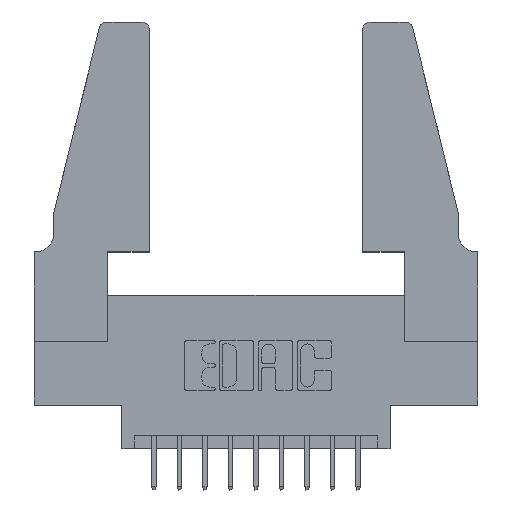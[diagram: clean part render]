
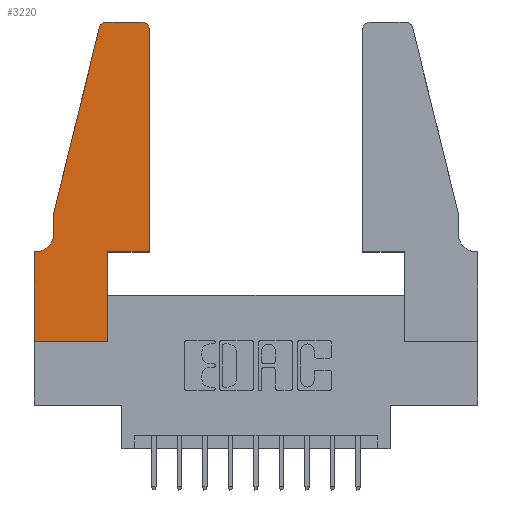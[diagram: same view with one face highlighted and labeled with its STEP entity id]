
A CAD part, top view. The second image highlights one B-rep face of the part: STEP entity #3220.
In plain terms, the highlighted planar face has unit normal (0, 0, 1).
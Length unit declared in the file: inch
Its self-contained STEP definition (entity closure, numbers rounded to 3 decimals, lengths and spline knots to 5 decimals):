
#200 = DIRECTION ( 'NONE',  ( 1., 0., 0. ) ) ;
#277 = VERTEX_POINT ( 'NONE', #6747 ) ;
#417 = LINE ( 'NONE', #4542, #11494 ) ;
#638 = CARTESIAN_POINT ( 'NONE',  ( 0.284, 1.25, 0.37 ) ) ;
#674 = VERTEX_POINT ( 'NONE', #3287 ) ;
#697 = EDGE_CURVE ( 'NONE', #674, #277, #417, .T. ) ;
#791 = DIRECTION ( 'NONE',  ( 1., 0., 0. ) ) ;
#899 = EDGE_CURVE ( 'NONE', #1029, #11434, #8804, .T. ) ;
#903 = CARTESIAN_POINT ( 'NONE',  ( 0.4205, 1.25, 0.37 ) ) ;
#1025 = DIRECTION ( 'NONE',  ( 0., 0., 1. ) ) ;
#1029 = VERTEX_POINT ( 'NONE', #6420 ) ;
#1111 = AXIS2_PLACEMENT_3D ( 'NONE', #13665, #13468, #5983 ) ;
#1183 = ORIENTED_EDGE ( 'NONE', *, *, #4739, .T. ) ;
#1201 = ORIENTED_EDGE ( 'NONE', *, *, #9031, .T. ) ;
#1419 = VECTOR ( 'NONE', #8248, 39.37008 ) ;
#1561 = EDGE_CURVE ( 'NONE', #5994, #674, #5780, .T. ) ;
#1776 = CARTESIAN_POINT ( 'NONE',  ( 0.4505, 0.35, 0.37 ) ) ;
#1813 = CARTESIAN_POINT ( 'NONE',  ( 0.2865, 0.35, 0.37 ) ) ;
#1864 = DIRECTION ( 'NONE',  ( 1., 0., 0. ) ) ;
#2030 = ORIENTED_EDGE ( 'NONE', *, *, #11785, .T. ) ;
#2249 = CARTESIAN_POINT ( 'NONE',  ( 0.284, 1.22, 0.37 ) ) ;
#2263 = CARTESIAN_POINT ( 'NONE',  ( 0.0755, 0.5, 0.37 ) ) ;
#2350 = CARTESIAN_POINT ( 'NONE',  ( 0., 0., 0.37 ) ) ;
#2599 = VECTOR ( 'NONE', #791, 39.37008 ) ;
#2892 = VECTOR ( 'NONE', #11044, 39.37008 ) ;
#2911 = ORIENTED_EDGE ( 'NONE', *, *, #1561, .T. ) ;
#3055 = EDGE_CURVE ( 'NONE', #13741, #5382, #11149, .T. ) ;
#3220 = ADVANCED_FACE ( 'NONE', ( #8140 ), #6419, .T. ) ;
#3287 = CARTESIAN_POINT ( 'NONE',  ( 0., 0.35, 0.37 ) ) ;
#3432 = LINE ( 'NONE', #2263, #13652 ) ;
#3437 = AXIS2_PLACEMENT_3D ( 'NONE', #12783, #1025, #6462 ) ;
#3440 = LINE ( 'NONE', #1813, #1419 ) ;
#3792 = ORIENTED_EDGE ( 'NONE', *, *, #697, .T. ) ;
#3890 = CARTESIAN_POINT ( 'NONE',  ( 0.4505, 1.22, 0.37 ) ) ;
#4404 = CARTESIAN_POINT ( 'NONE',  ( 0.0755, 0.5, 0.37 ) ) ;
#4542 = CARTESIAN_POINT ( 'NONE',  ( 0., 0., 0.37 ) ) ;
#4690 = CARTESIAN_POINT ( 'NONE',  ( 0.25487, 1.22718, 0.37 ) ) ;
#4714 = CARTESIAN_POINT ( 'NONE',  ( 0.2865, 0., 0.37 ) ) ;
#4722 = VERTEX_POINT ( 'NONE', #903 ) ;
#4739 = EDGE_CURVE ( 'NONE', #8224, #5994, #10923, .T. ) ;
#4751 = CARTESIAN_POINT ( 'NONE',  ( 0.0755, 0.35, 0.37 ) ) ;
#5096 = ORIENTED_EDGE ( 'NONE', *, *, #7326, .T. ) ;
#5260 = VECTOR ( 'NONE', #10212, 39.37008 ) ;
#5294 = VERTEX_POINT ( 'NONE', #638 ) ;
#5382 = VERTEX_POINT ( 'NONE', #6079 ) ;
#5386 = ORIENTED_EDGE ( 'NONE', *, *, #8547, .T. ) ;
#5539 = DIRECTION ( 'NONE',  ( 0., -1., 0. ) ) ;
#5780 = LINE ( 'NONE', #4751, #5260 ) ;
#5925 = CARTESIAN_POINT ( 'NONE',  ( 0.0055, 0.35, 0.37 ) ) ;
#5983 = DIRECTION ( 'NONE',  ( -1., 0., 0. ) ) ;
#5994 = VERTEX_POINT ( 'NONE', #5925 ) ;
#6079 = CARTESIAN_POINT ( 'NONE',  ( 0.0755, 0.5, 0.37 ) ) ;
#6184 = VERTEX_POINT ( 'NONE', #4714 ) ;
#6419 = PLANE ( 'NONE',  #3437 ) ;
#6420 = CARTESIAN_POINT ( 'NONE',  ( 0.2865, 0.35, 0.37 ) ) ;
#6462 = DIRECTION ( 'NONE',  ( 1., 0., 0. ) ) ;
#6649 = DIRECTION ( 'NONE',  ( 1., 0., 0. ) ) ;
#6671 = ORIENTED_EDGE ( 'NONE', *, *, #13728, .T. ) ;
#6747 = CARTESIAN_POINT ( 'NONE',  ( 0., 0., 0.37 ) ) ;
#6778 = CIRCLE ( 'NONE', #12624, 0.03 ) ;
#6855 = ORIENTED_EDGE ( 'NONE', *, *, #8538, .T. ) ;
#7132 = CARTESIAN_POINT ( 'NONE',  ( 0.4505, 0.35, 0.37 ) ) ;
#7326 = EDGE_CURVE ( 'NONE', #277, #6184, #10505, .T. ) ;
#7812 = CARTESIAN_POINT ( 'NONE',  ( 0.2605, 1.25, 0.37 ) ) ;
#8060 = ORIENTED_EDGE ( 'NONE', *, *, #899, .T. ) ;
#8140 = FACE_OUTER_BOUND ( 'NONE', #9539, .T. ) ;
#8224 = VERTEX_POINT ( 'NONE', #9288 ) ;
#8248 = DIRECTION ( 'NONE',  ( 0., 1., 0. ) ) ;
#8538 = EDGE_CURVE ( 'NONE', #13219, #4722, #6778, .T. ) ;
#8547 = EDGE_CURVE ( 'NONE', #6184, #1029, #3440, .T. ) ;
#8804 = LINE ( 'NONE', #1776, #2599 ) ;
#8843 = AXIS2_PLACEMENT_3D ( 'NONE', #2249, #9776, #6649 ) ;
#9017 = VECTOR ( 'NONE', #13246, 39.37008 ) ;
#9031 = EDGE_CURVE ( 'NONE', #5382, #8224, #3432, .T. ) ;
#9288 = CARTESIAN_POINT ( 'NONE',  ( 0.0755, 0.42, 0.37 ) ) ;
#9539 = EDGE_LOOP ( 'NONE', ( #13878, #2030, #12322, #1201, #1183, #2911, #3792, #5096, #5386, #8060, #6671, #6855 ) ) ;
#9776 = DIRECTION ( 'NONE',  ( 0., 0., 1. ) ) ;
#9866 = DIRECTION ( 'NONE',  ( -0.239, -0.971, 0. ) ) ;
#10008 = EDGE_CURVE ( 'NONE', #4722, #5294, #12946, .T. ) ;
#10212 = DIRECTION ( 'NONE',  ( -1., 0., 0. ) ) ;
#10332 = DIRECTION ( 'NONE',  ( 0., 0., 1. ) ) ;
#10505 = LINE ( 'NONE', #2350, #11703 ) ;
#10923 = CIRCLE ( 'NONE', #1111, 0.07 ) ;
#11044 = DIRECTION ( 'NONE',  ( -1., 0., 0. ) ) ;
#11112 = CARTESIAN_POINT ( 'NONE',  ( 0.4505, 0.35, 0.37 ) ) ;
#11149 = LINE ( 'NONE', #4404, #11979 ) ;
#11255 = CIRCLE ( 'NONE', #8843, 0.03 ) ;
#11434 = VERTEX_POINT ( 'NONE', #7132 ) ;
#11494 = VECTOR ( 'NONE', #12024, 39.37008 ) ;
#11703 = VECTOR ( 'NONE', #200, 39.37008 ) ;
#11785 = EDGE_CURVE ( 'NONE', #5294, #13741, #11255, .T. ) ;
#11979 = VECTOR ( 'NONE', #9866, 39.37008 ) ;
#12024 = DIRECTION ( 'NONE',  ( 0., -1., 0. ) ) ;
#12026 = LINE ( 'NONE', #11112, #9017 ) ;
#12322 = ORIENTED_EDGE ( 'NONE', *, *, #3055, .T. ) ;
#12450 = CARTESIAN_POINT ( 'NONE',  ( 0.4205, 1.22, 0.37 ) ) ;
#12624 = AXIS2_PLACEMENT_3D ( 'NONE', #12450, #10332, #1864 ) ;
#12783 = CARTESIAN_POINT ( 'NONE',  ( 0., 0.35, 0.37 ) ) ;
#12946 = LINE ( 'NONE', #7812, #2892 ) ;
#13219 = VERTEX_POINT ( 'NONE', #3890 ) ;
#13246 = DIRECTION ( 'NONE',  ( 0., 1., 0. ) ) ;
#13468 = DIRECTION ( 'NONE',  ( 0., 0., -1. ) ) ;
#13652 = VECTOR ( 'NONE', #5539, 39.37008 ) ;
#13665 = CARTESIAN_POINT ( 'NONE',  ( 0.0055, 0.42, 0.37 ) ) ;
#13728 = EDGE_CURVE ( 'NONE', #11434, #13219, #12026, .T. ) ;
#13741 = VERTEX_POINT ( 'NONE', #4690 ) ;
#13878 = ORIENTED_EDGE ( 'NONE', *, *, #10008, .T. ) ;
